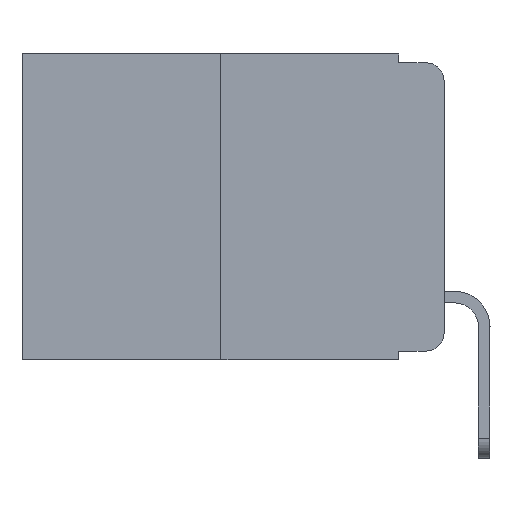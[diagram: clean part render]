
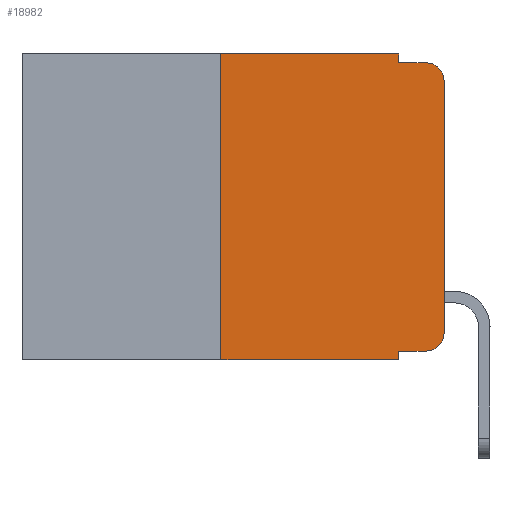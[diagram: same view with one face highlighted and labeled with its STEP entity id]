
A CAD part, left-side view. The second image highlights one B-rep face of the part: STEP entity #18982.
In plain terms, the highlighted planar face has unit normal (-1, 0, 0).
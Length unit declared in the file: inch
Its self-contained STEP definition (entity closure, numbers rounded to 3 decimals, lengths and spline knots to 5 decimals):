
#13 = EDGE_CURVE ( 'NONE', #17101, #11079, #23737, .T. ) ;
#336 = CARTESIAN_POINT ( 'NONE',  ( 0., 0.25, -0.343 ) ) ;
#641 = DIRECTION ( 'NONE',  ( 0., 0., 1. ) ) ;
#816 = VECTOR ( 'NONE', #15919, 39.37008 ) ;
#1456 = CARTESIAN_POINT ( 'NONE',  ( 0., 0.051, 0. ) ) ;
#1560 = LINE ( 'NONE', #7815, #6541 ) ;
#1699 = LINE ( 'NONE', #22099, #6658 ) ;
#2241 = VERTEX_POINT ( 'NONE', #24089 ) ;
#3834 = CARTESIAN_POINT ( 'NONE',  ( 0., 0.25, 0. ) ) ;
#4262 = CARTESIAN_POINT ( 'NONE',  ( 0., 0., -0.313 ) ) ;
#4771 = CARTESIAN_POINT ( 'NONE',  ( 0., 0.02, -0.333 ) ) ;
#5812 = CARTESIAN_POINT ( 'NONE',  ( 0., 0.051, -0.01 ) ) ;
#6107 = CARTESIAN_POINT ( 'NONE',  ( 0., 0.051, -0.333 ) ) ;
#6204 = LINE ( 'NONE', #11201, #11004 ) ;
#6318 = VERTEX_POINT ( 'NONE', #11168 ) ;
#6541 = VECTOR ( 'NONE', #15769, 39.37008 ) ;
#6624 = VERTEX_POINT ( 'NONE', #8116 ) ;
#6658 = VECTOR ( 'NONE', #12266, 39.37008 ) ;
#6874 = CARTESIAN_POINT ( 'NONE',  ( 0., 0.473, 0. ) ) ;
#7109 = CARTESIAN_POINT ( 'NONE',  ( 0., 0.051, -0.01 ) ) ;
#7112 = EDGE_CURVE ( 'NONE', #20068, #17101, #1560, .T. ) ;
#7359 = CARTESIAN_POINT ( 'NONE',  ( 0., 0.473, 0. ) ) ;
#7480 = FACE_OUTER_BOUND ( 'NONE', #12670, .T. ) ;
#7815 = CARTESIAN_POINT ( 'NONE',  ( 0., 0.051, -0.333 ) ) ;
#7893 = ORIENTED_EDGE ( 'NONE', *, *, #14326, .F. ) ;
#8116 = CARTESIAN_POINT ( 'NONE',  ( 0., 0., -0.03 ) ) ;
#8562 = ORIENTED_EDGE ( 'NONE', *, *, #17791, .T. ) ;
#8932 = LINE ( 'NONE', #3834, #9560 ) ;
#9016 = CARTESIAN_POINT ( 'NONE',  ( 0., 0., 0. ) ) ;
#9041 = DIRECTION ( 'NONE',  ( 1., 0., 0. ) ) ;
#9264 = CARTESIAN_POINT ( 'NONE',  ( 0., 0.02, -0.03 ) ) ;
#9560 = VECTOR ( 'NONE', #17977, 39.37008 ) ;
#11004 = VECTOR ( 'NONE', #20657, 39.37008 ) ;
#11079 = VERTEX_POINT ( 'NONE', #4262 ) ;
#11168 = CARTESIAN_POINT ( 'NONE',  ( 0., 0.25, 0. ) ) ;
#11201 = CARTESIAN_POINT ( 'NONE',  ( 0., 0.473, -0.343 ) ) ;
#11353 = DIRECTION ( 'NONE',  ( 0., 0., -1. ) ) ;
#11587 = AXIS2_PLACEMENT_3D ( 'NONE', #9264, #23203, #11353 ) ;
#11787 = ORIENTED_EDGE ( 'NONE', *, *, #15664, .F. ) ;
#12266 = DIRECTION ( 'NONE',  ( 0., 0., -1. ) ) ;
#12526 = EDGE_CURVE ( 'NONE', #6624, #26303, #24835, .T. ) ;
#12670 = EDGE_LOOP ( 'NONE', ( #8562, #19201, #14604, #25687, #26320, #11787, #22586, #7893, #13929, #19820 ) ) ;
#13367 = CARTESIAN_POINT ( 'NONE',  ( 0., 0.02, -0.313 ) ) ;
#13660 = VERTEX_POINT ( 'NONE', #16006 ) ;
#13929 = ORIENTED_EDGE ( 'NONE', *, *, #7112, .T. ) ;
#14326 = EDGE_CURVE ( 'NONE', #20068, #13660, #1699, .T. ) ;
#14557 = VECTOR ( 'NONE', #641, 39.37008 ) ;
#14604 = ORIENTED_EDGE ( 'NONE', *, *, #23568, .F. ) ;
#15326 = VECTOR ( 'NONE', #15772, 39.37008 ) ;
#15446 = AXIS2_PLACEMENT_3D ( 'NONE', #6874, #9041, #22969 ) ;
#15554 = LINE ( 'NONE', #7359, #20204 ) ;
#15664 = EDGE_CURVE ( 'NONE', #24381, #6318, #8932, .T. ) ;
#15769 = DIRECTION ( 'NONE',  ( 0., -1., 0. ) ) ;
#15772 = DIRECTION ( 'NONE',  ( 0., 0., -1. ) ) ;
#15919 = DIRECTION ( 'NONE',  ( 0., -1., 0. ) ) ;
#16006 = CARTESIAN_POINT ( 'NONE',  ( 0., 0.051, -0.343 ) ) ;
#16618 = LINE ( 'NONE', #5812, #816 ) ;
#17101 = VERTEX_POINT ( 'NONE', #4771 ) ;
#17579 = CARTESIAN_POINT ( 'NONE',  ( 0., 0.02, -0.01 ) ) ;
#17791 = EDGE_CURVE ( 'NONE', #11079, #6624, #19799, .T. ) ;
#17847 = VERTEX_POINT ( 'NONE', #7109 ) ;
#17977 = DIRECTION ( 'NONE',  ( 0., 0., 1. ) ) ;
#18982 = ADVANCED_FACE ( 'NONE', ( #7480 ), #21022, .F. ) ;
#19039 = EDGE_CURVE ( 'NONE', #24381, #13660, #6204, .T. ) ;
#19201 = ORIENTED_EDGE ( 'NONE', *, *, #12526, .T. ) ;
#19394 = DIRECTION ( 'NONE',  ( 0., -1., 0. ) ) ;
#19799 = LINE ( 'NONE', #9016, #14557 ) ;
#19820 = ORIENTED_EDGE ( 'NONE', *, *, #13, .T. ) ;
#20068 = VERTEX_POINT ( 'NONE', #6107 ) ;
#20204 = VECTOR ( 'NONE', #19394, 39.37008 ) ;
#20657 = DIRECTION ( 'NONE',  ( 0., -1., 0. ) ) ;
#21022 = PLANE ( 'NONE',  #15446 ) ;
#21580 = DIRECTION ( 'NONE',  ( 0., 0., -1. ) ) ;
#21660 = DIRECTION ( 'NONE',  ( -1., 0., 0. ) ) ;
#22099 = CARTESIAN_POINT ( 'NONE',  ( 0., 0.051, 0. ) ) ;
#22140 = EDGE_CURVE ( 'NONE', #6318, #2241, #15554, .T. ) ;
#22262 = EDGE_CURVE ( 'NONE', #2241, #17847, #22331, .T. ) ;
#22331 = LINE ( 'NONE', #1456, #15326 ) ;
#22586 = ORIENTED_EDGE ( 'NONE', *, *, #19039, .T. ) ;
#22969 = DIRECTION ( 'NONE',  ( 0., 0., -1. ) ) ;
#23203 = DIRECTION ( 'NONE',  ( -1., 0., 0. ) ) ;
#23481 = AXIS2_PLACEMENT_3D ( 'NONE', #13367, #21660, #21580 ) ;
#23568 = EDGE_CURVE ( 'NONE', #17847, #26303, #16618, .T. ) ;
#23737 = CIRCLE ( 'NONE', #23481, 0.02 ) ;
#24089 = CARTESIAN_POINT ( 'NONE',  ( 0., 0.051, 0. ) ) ;
#24381 = VERTEX_POINT ( 'NONE', #336 ) ;
#24835 = CIRCLE ( 'NONE', #11587, 0.02 ) ;
#25687 = ORIENTED_EDGE ( 'NONE', *, *, #22262, .F. ) ;
#26303 = VERTEX_POINT ( 'NONE', #17579 ) ;
#26320 = ORIENTED_EDGE ( 'NONE', *, *, #22140, .F. ) ;
